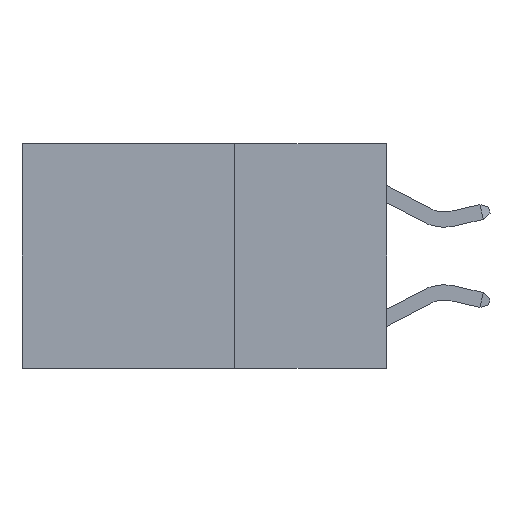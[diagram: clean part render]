
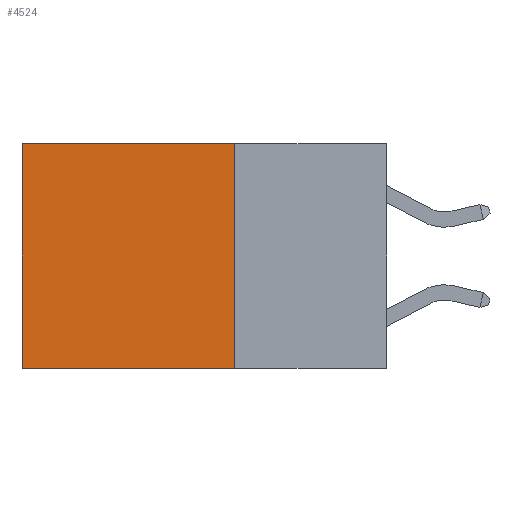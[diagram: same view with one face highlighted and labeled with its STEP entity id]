
A CAD part, left-side view. The second image highlights one B-rep face of the part: STEP entity #4524.
In plain terms, the highlighted planar face has unit normal (-1, 0, 0).
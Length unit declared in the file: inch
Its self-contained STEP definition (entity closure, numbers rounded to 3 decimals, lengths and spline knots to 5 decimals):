
#137 = ORIENTED_EDGE ( 'NONE', *, *, #5951, .F. ) ;
#198 = VECTOR ( 'NONE', #9428, 39.37008 ) ;
#247 = CARTESIAN_POINT ( 'NONE',  ( 0.2625, 0.6, -0.37 ) ) ;
#365 = DIRECTION ( 'NONE',  ( 0., 0., -1. ) ) ;
#849 = DIRECTION ( 'NONE',  ( 0., 1., 0. ) ) ;
#1655 = EDGE_LOOP ( 'NONE', ( #8429, #137, #2090, #8739 ) ) ;
#1925 = PLANE ( 'NONE',  #5073 ) ;
#2090 = ORIENTED_EDGE ( 'NONE', *, *, #4119, .F. ) ;
#2748 = VECTOR ( 'NONE', #7085, 39.37008 ) ;
#2935 = CARTESIAN_POINT ( 'NONE',  ( 0.2625, 0.25, 0. ) ) ;
#3072 = CARTESIAN_POINT ( 'NONE',  ( 0.2625, 0.6, 0. ) ) ;
#3074 = FACE_OUTER_BOUND ( 'NONE', #1655, .T. ) ;
#3682 = DIRECTION ( 'NONE',  ( 0., 0., -1. ) ) ;
#4119 = EDGE_CURVE ( 'NONE', #8620, #7559, #8260, .T. ) ;
#4524 = ADVANCED_FACE ( 'NONE', ( #3074 ), #1925, .F. ) ;
#5003 = EDGE_CURVE ( 'NONE', #8885, #6101, #9042, .T. ) ;
#5073 = AXIS2_PLACEMENT_3D ( 'NONE', #7728, #8474, #3682 ) ;
#5262 = LINE ( 'NONE', #6858, #7172 ) ;
#5275 = LINE ( 'NONE', #2935, #2748 ) ;
#5564 = CARTESIAN_POINT ( 'NONE',  ( 0.2625, 0.6, 0. ) ) ;
#5613 = CARTESIAN_POINT ( 'NONE',  ( 0.2625, 0.25, 0. ) ) ;
#5630 = EDGE_CURVE ( 'NONE', #8620, #8885, #5275, .T. ) ;
#5951 = EDGE_CURVE ( 'NONE', #7559, #6101, #5262, .T. ) ;
#6101 = VERTEX_POINT ( 'NONE', #247 ) ;
#6515 = VECTOR ( 'NONE', #365, 39.37008 ) ;
#6576 = CARTESIAN_POINT ( 'NONE',  ( 0.2625, 0.25, -0.37 ) ) ;
#6858 = CARTESIAN_POINT ( 'NONE',  ( 0.2625, 0.25, -0.37 ) ) ;
#7085 = DIRECTION ( 'NONE',  ( 0., 1., 0. ) ) ;
#7172 = VECTOR ( 'NONE', #849, 39.37008 ) ;
#7559 = VERTEX_POINT ( 'NONE', #6576 ) ;
#7728 = CARTESIAN_POINT ( 'NONE',  ( 0.2625, 0.25, 0. ) ) ;
#8260 = LINE ( 'NONE', #5613, #6515 ) ;
#8429 = ORIENTED_EDGE ( 'NONE', *, *, #5003, .T. ) ;
#8474 = DIRECTION ( 'NONE',  ( 1., 0., 0. ) ) ;
#8620 = VERTEX_POINT ( 'NONE', #10394 ) ;
#8739 = ORIENTED_EDGE ( 'NONE', *, *, #5630, .T. ) ;
#8885 = VERTEX_POINT ( 'NONE', #5564 ) ;
#9042 = LINE ( 'NONE', #3072, #198 ) ;
#9428 = DIRECTION ( 'NONE',  ( 0., 0., -1. ) ) ;
#10394 = CARTESIAN_POINT ( 'NONE',  ( 0.2625, 0.25, 0. ) ) ;
